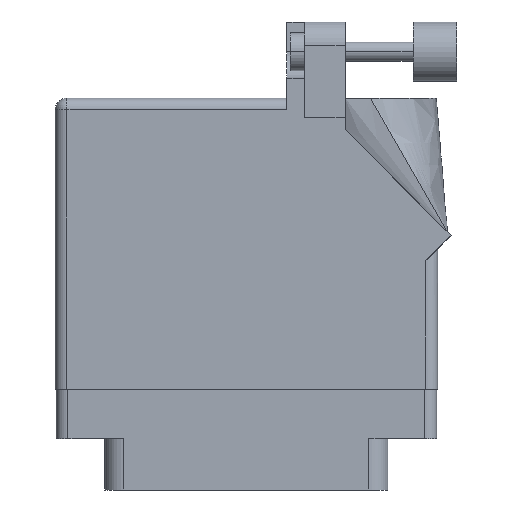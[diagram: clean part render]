
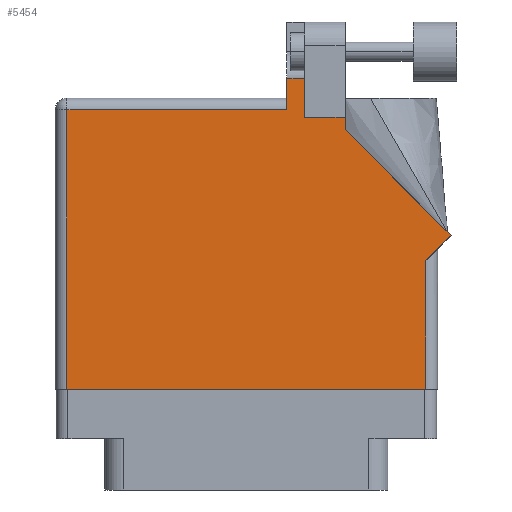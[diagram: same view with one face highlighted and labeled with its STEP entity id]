
A CAD part, front view. The second image highlights one B-rep face of the part: STEP entity #5454.
In plain terms, the highlighted face is planar.
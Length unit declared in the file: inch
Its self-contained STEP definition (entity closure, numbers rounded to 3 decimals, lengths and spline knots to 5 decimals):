
#513 = ORIENTED_EDGE ( 'NONE', *, *, #20524, .T. ) ;
#856 = LINE ( 'NONE', #6397, #24596 ) ;
#860 = VERTEX_POINT ( 'NONE', #26351 ) ;
#1615 = DIRECTION ( 'NONE',  ( 0.707, 0.707, 0. ) ) ;
#2106 = CARTESIAN_POINT ( 'NONE',  ( 1.948, 0., 0. ) ) ;
#2700 = DIRECTION ( 'NONE',  ( 0., 0., -1. ) ) ;
#2792 = VERTEX_POINT ( 'NONE', #38399 ) ;
#2916 = CARTESIAN_POINT ( 'NONE',  ( 2.08071, 0.80771, 0. ) ) ;
#3894 = ORIENTED_EDGE ( 'NONE', *, *, #30955, .T. ) ;
#4442 = LINE ( 'NONE', #15197, #25357 ) ;
#4978 = CARTESIAN_POINT ( 'NONE',  ( 1.217, 1.6315, 0. ) ) ;
#5350 = CARTESIAN_POINT ( 'NONE',  ( 0., 1.53, 0. ) ) ;
#5400 = CARTESIAN_POINT ( 'NONE',  ( 1.217, 1.53, 0. ) ) ;
#5454 = ADVANCED_FACE ( 'NONE', ( #6722 ), #21035, .F. ) ;
#5567 = EDGE_CURVE ( 'NONE', #19321, #32012, #22928, .T. ) ;
#5774 = VERTEX_POINT ( 'NONE', #16279 ) ;
#5911 = LINE ( 'NONE', #25294, #38690 ) ;
#6034 = DIRECTION ( 'NONE',  ( -1., 0., 0. ) ) ;
#6397 = CARTESIAN_POINT ( 'NONE',  ( 0., 0., 0. ) ) ;
#6699 = LINE ( 'NONE', #16404, #10035 ) ;
#6722 = FACE_OUTER_BOUND ( 'NONE', #7010, .T. ) ;
#7003 = EDGE_CURVE ( 'NONE', #31177, #30890, #4442, .T. ) ;
#7010 = EDGE_LOOP ( 'NONE', ( #29856, #20686, #28555, #15108, #3894, #10562, #513, #10940, #28287, #13414, #17540 ) ) ;
#8140 = DIRECTION ( 'NONE',  ( 0., -1., 0. ) ) ;
#8165 = EDGE_CURVE ( 'NONE', #11515, #5774, #6699, .T. ) ;
#9214 = EDGE_CURVE ( 'NONE', #860, #19321, #9449, .T. ) ;
#9301 = LINE ( 'NONE', #26617, #30317 ) ;
#9404 = VECTOR ( 'NONE', #8140, 39.37008 ) ;
#9449 = LINE ( 'NONE', #13364, #31904 ) ;
#9486 = VECTOR ( 'NONE', #17723, 39.37008 ) ;
#10007 = AXIS2_PLACEMENT_3D ( 'NONE', #5350, #2700, #38811 ) ;
#10035 = VECTOR ( 'NONE', #37695, 39.37008 ) ;
#10440 = VERTEX_POINT ( 'NONE', #37649 ) ;
#10562 = ORIENTED_EDGE ( 'NONE', *, *, #11244, .T. ) ;
#10863 = DIRECTION ( 'NONE',  ( -0.707, 0.707, 0. ) ) ;
#10940 = ORIENTED_EDGE ( 'NONE', *, *, #9214, .T. ) ;
#11244 = EDGE_CURVE ( 'NONE', #10440, #29814, #856, .T. ) ;
#11515 = VERTEX_POINT ( 'NONE', #35381 ) ;
#11578 = EDGE_CURVE ( 'NONE', #32012, #2792, #9301, .T. ) ;
#12688 = DIRECTION ( 'NONE',  ( -1., 0., 0. ) ) ;
#12739 = DIRECTION ( 'NONE',  ( 1., 0., 0. ) ) ;
#13364 = CARTESIAN_POINT ( 'NONE',  ( 2.01, 0.737, 0. ) ) ;
#13414 = ORIENTED_EDGE ( 'NONE', *, *, #11578, .T. ) ;
#15086 = DIRECTION ( 'NONE',  ( -1., 0., 0. ) ) ;
#15108 = ORIENTED_EDGE ( 'NONE', *, *, #7003, .T. ) ;
#15197 = CARTESIAN_POINT ( 'NONE',  ( 0., 1.468, 0. ) ) ;
#16242 = CARTESIAN_POINT ( 'NONE',  ( 0.062, 1.468, 0. ) ) ;
#16279 = CARTESIAN_POINT ( 'NONE',  ( 1.311, 1.6315, 0. ) ) ;
#16404 = CARTESIAN_POINT ( 'NONE',  ( 1.311, 1.43, 0. ) ) ;
#16649 = LINE ( 'NONE', #5400, #9486 ) ;
#17540 = ORIENTED_EDGE ( 'NONE', *, *, #21390, .T. ) ;
#17723 = DIRECTION ( 'NONE',  ( 0., -1., 0. ) ) ;
#19321 = VERTEX_POINT ( 'NONE', #22317 ) ;
#20485 = DIRECTION ( 'NONE',  ( 0., 1., 0. ) ) ;
#20524 = EDGE_CURVE ( 'NONE', #29814, #860, #5911, .T. ) ;
#20686 = ORIENTED_EDGE ( 'NONE', *, *, #23427, .T. ) ;
#21035 = PLANE ( 'NONE',  #10007 ) ;
#21390 = EDGE_CURVE ( 'NONE', #2792, #11515, #24348, .T. ) ;
#22317 = CARTESIAN_POINT ( 'NONE',  ( 2.08071, 0.80771, 0. ) ) ;
#22455 = VECTOR ( 'NONE', #15086, 39.37008 ) ;
#22738 = EDGE_CURVE ( 'NONE', #31054, #31177, #16649, .T. ) ;
#22928 = LINE ( 'NONE', #2916, #29141 ) ;
#23282 = VECTOR ( 'NONE', #6034, 39.37008 ) ;
#23427 = EDGE_CURVE ( 'NONE', #5774, #31054, #27589, .T. ) ;
#24106 = CARTESIAN_POINT ( 'NONE',  ( 1.64177, 1.6315, 0. ) ) ;
#24256 = CARTESIAN_POINT ( 'NONE',  ( 1.524, 1.43, 0. ) ) ;
#24348 = LINE ( 'NONE', #24256, #22455 ) ;
#24596 = VECTOR ( 'NONE', #12739, 39.37008 ) ;
#25294 = CARTESIAN_POINT ( 'NONE',  ( 1.948, 0.737, 0. ) ) ;
#25357 = VECTOR ( 'NONE', #12688, 39.37008 ) ;
#26351 = CARTESIAN_POINT ( 'NONE',  ( 1.948, 0.675, 0. ) ) ;
#26615 = LINE ( 'NONE', #35037, #9404 ) ;
#26617 = CARTESIAN_POINT ( 'NONE',  ( 1.524, 1.36442, 0. ) ) ;
#27589 = LINE ( 'NONE', #24106, #23282 ) ;
#28287 = ORIENTED_EDGE ( 'NONE', *, *, #5567, .T. ) ;
#28555 = ORIENTED_EDGE ( 'NONE', *, *, #22738, .T. ) ;
#29141 = VECTOR ( 'NONE', #10863, 39.37008 ) ;
#29814 = VERTEX_POINT ( 'NONE', #2106 ) ;
#29856 = ORIENTED_EDGE ( 'NONE', *, *, #8165, .T. ) ;
#30317 = VECTOR ( 'NONE', #20485, 39.37008 ) ;
#30890 = VERTEX_POINT ( 'NONE', #16242 ) ;
#30955 = EDGE_CURVE ( 'NONE', #30890, #10440, #26615, .T. ) ;
#31054 = VERTEX_POINT ( 'NONE', #4978 ) ;
#31177 = VERTEX_POINT ( 'NONE', #33138 ) ;
#31719 = DIRECTION ( 'NONE',  ( 0., 1., 0. ) ) ;
#31904 = VECTOR ( 'NONE', #1615, 39.37008 ) ;
#32012 = VERTEX_POINT ( 'NONE', #33954 ) ;
#33138 = CARTESIAN_POINT ( 'NONE',  ( 1.217, 1.468, 0. ) ) ;
#33954 = CARTESIAN_POINT ( 'NONE',  ( 1.524, 1.36442, 0. ) ) ;
#35037 = CARTESIAN_POINT ( 'NONE',  ( 0.062, 0., 0. ) ) ;
#35381 = CARTESIAN_POINT ( 'NONE',  ( 1.311, 1.43, 0. ) ) ;
#37649 = CARTESIAN_POINT ( 'NONE',  ( 0.062, 0., 0. ) ) ;
#37695 = DIRECTION ( 'NONE',  ( 0., 1., 0. ) ) ;
#38399 = CARTESIAN_POINT ( 'NONE',  ( 1.524, 1.43, 0. ) ) ;
#38690 = VECTOR ( 'NONE', #31719, 39.37008 ) ;
#38811 = DIRECTION ( 'NONE',  ( -1., 0., 0. ) ) ;
